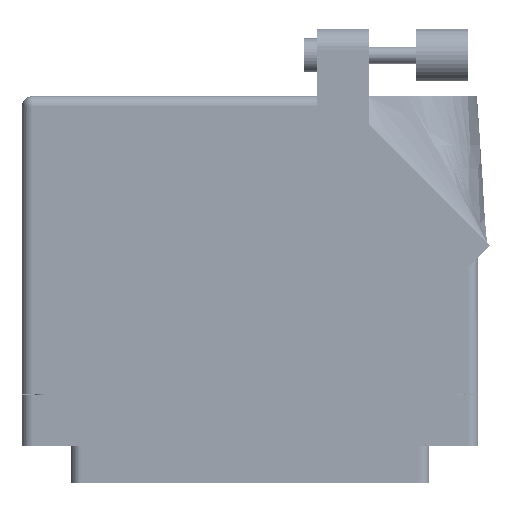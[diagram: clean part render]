
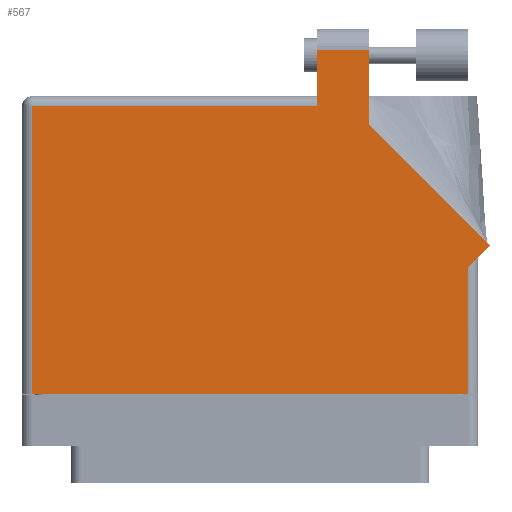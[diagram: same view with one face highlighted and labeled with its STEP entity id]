
A CAD part, front view. The second image highlights one B-rep face of the part: STEP entity #567.
In plain terms, the highlighted face is planar.
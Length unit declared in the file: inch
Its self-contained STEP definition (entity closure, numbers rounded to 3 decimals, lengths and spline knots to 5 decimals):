
#553 = EDGE_CURVE ( 'NONE', #56019, #10716, #7325, .T. ) ;
#567 = ADVANCED_FACE ( 'NONE', ( #53684 ), #71045, .F. ) ;
#1830 = CARTESIAN_POINT ( 'NONE',  ( 1.42971, 0.78571, 0.617 ) ) ;
#5146 = CARTESIAN_POINT ( 'NONE',  ( -1.297, 1.613, 0.617 ) ) ;
#5155 = EDGE_LOOP ( 'NONE', ( #65231, #48399, #29454, #40733, #71744, #52647, #39767, #5816, #29157 ) ) ;
#5320 = VECTOR ( 'NONE', #65843, 39.37008 ) ;
#5524 = VERTEX_POINT ( 'NONE', #60224 ) ;
#5816 = ORIENTED_EDGE ( 'NONE', *, *, #23467, .T. ) ;
#6621 = EDGE_CURVE ( 'NONE', #67285, #56019, #48871, .T. ) ;
#7259 = CARTESIAN_POINT ( 'NONE',  ( -1.297, -0.1, 0.617 ) ) ;
#7325 = LINE ( 'NONE', #70539, #44837 ) ;
#9706 = VECTOR ( 'NONE', #67357, 39.37008 ) ;
#10716 = VERTEX_POINT ( 'NONE', #7259 ) ;
#12158 = DIRECTION ( 'NONE',  ( 1., 0., 0. ) ) ;
#12598 = DIRECTION ( 'NONE',  ( -0.707, 0.707, 0. ) ) ;
#14162 = DIRECTION ( 'NONE',  ( -1., 0., 0. ) ) ;
#14236 = CARTESIAN_POINT ( 'NONE',  ( -1.359, 1.675, 0.617 ) ) ;
#15503 = DIRECTION ( 'NONE',  ( 0., 0., -1. ) ) ;
#15565 = CARTESIAN_POINT ( 'NONE',  ( 0.399, 1.675, 0.617 ) ) ;
#20514 = LINE ( 'NONE', #59876, #5320 ) ;
#20780 = DIRECTION ( 'NONE',  ( 0., -1., 0. ) ) ;
#21946 = AXIS2_PLACEMENT_3D ( 'NONE', #14236, #15503, #73035 ) ;
#23467 = EDGE_CURVE ( 'NONE', #33412, #65912, #20514, .T. ) ;
#24420 = CARTESIAN_POINT ( 'NONE',  ( 1.297, -0.1, 0.617 ) ) ;
#25420 = LINE ( 'NONE', #1830, #34252 ) ;
#26134 = VERTEX_POINT ( 'NONE', #42292 ) ;
#28029 = VECTOR ( 'NONE', #14162, 39.37008 ) ;
#28233 = VECTOR ( 'NONE', #20780, 39.37008 ) ;
#28450 = LINE ( 'NONE', #52500, #62269 ) ;
#29157 = ORIENTED_EDGE ( 'NONE', *, *, #33405, .T. ) ;
#29357 = CARTESIAN_POINT ( 'NONE',  ( 0.706, 1.50942, 0.617 ) ) ;
#29454 = ORIENTED_EDGE ( 'NONE', *, *, #32032, .T. ) ;
#29729 = LINE ( 'NONE', #29357, #51129 ) ;
#31223 = DIRECTION ( 'NONE',  ( 0., -1., 0. ) ) ;
#32032 = EDGE_CURVE ( 'NONE', #44872, #67285, #62049, .T. ) ;
#32400 = CARTESIAN_POINT ( 'NONE',  ( 0.399, 1.613, 0.617 ) ) ;
#32910 = LINE ( 'NONE', #45788, #48856 ) ;
#33076 = CARTESIAN_POINT ( 'NONE',  ( 1.42971, 0.78571, 0.617 ) ) ;
#33405 = EDGE_CURVE ( 'NONE', #65912, #26134, #25420, .T. ) ;
#33412 = VERTEX_POINT ( 'NONE', #70382 ) ;
#33787 = CARTESIAN_POINT ( 'NONE',  ( -1.359, 1.613, 0.617 ) ) ;
#34252 = VECTOR ( 'NONE', #12598, 39.37008 ) ;
#34839 = DIRECTION ( 'NONE',  ( 0., 1., 0. ) ) ;
#36847 = EDGE_CURVE ( 'NONE', #63888, #33412, #28450, .T. ) ;
#39032 = EDGE_CURVE ( 'NONE', #10716, #63888, #32910, .T. ) ;
#39767 = ORIENTED_EDGE ( 'NONE', *, *, #36847, .T. ) ;
#40076 = CARTESIAN_POINT ( 'NONE',  ( 0.399, 1.95, 0.617 ) ) ;
#40733 = ORIENTED_EDGE ( 'NONE', *, *, #6621, .T. ) ;
#42292 = CARTESIAN_POINT ( 'NONE',  ( 0.706, 1.50942, 0.617 ) ) ;
#44083 = LINE ( 'NONE', #54230, #28029 ) ;
#44837 = VECTOR ( 'NONE', #31223, 39.37008 ) ;
#44872 = VERTEX_POINT ( 'NONE', #40076 ) ;
#45788 = CARTESIAN_POINT ( 'NONE',  ( -1.359, -0.1, 0.617 ) ) ;
#46879 = EDGE_CURVE ( 'NONE', #5524, #44872, #44083, .T. ) ;
#47125 = EDGE_CURVE ( 'NONE', #26134, #5524, #29729, .T. ) ;
#48399 = ORIENTED_EDGE ( 'NONE', *, *, #46879, .T. ) ;
#48856 = VECTOR ( 'NONE', #12158, 39.37008 ) ;
#48871 = LINE ( 'NONE', #33787, #9706 ) ;
#51129 = VECTOR ( 'NONE', #34839, 39.37008 ) ;
#52500 = CARTESIAN_POINT ( 'NONE',  ( 1.297, 0.715, 0.617 ) ) ;
#52647 = ORIENTED_EDGE ( 'NONE', *, *, #39032, .T. ) ;
#53254 = DIRECTION ( 'NONE',  ( 0., 1., 0. ) ) ;
#53684 = FACE_OUTER_BOUND ( 'NONE', #5155, .T. ) ;
#54230 = CARTESIAN_POINT ( 'NONE',  ( 0.399, 1.95, 0.617 ) ) ;
#56019 = VERTEX_POINT ( 'NONE', #5146 ) ;
#59876 = CARTESIAN_POINT ( 'NONE',  ( 1.359, 0.715, 0.617 ) ) ;
#60224 = CARTESIAN_POINT ( 'NONE',  ( 0.706, 1.95, 0.617 ) ) ;
#62049 = LINE ( 'NONE', #15565, #28233 ) ;
#62269 = VECTOR ( 'NONE', #53254, 39.37008 ) ;
#63888 = VERTEX_POINT ( 'NONE', #24420 ) ;
#65231 = ORIENTED_EDGE ( 'NONE', *, *, #47125, .T. ) ;
#65843 = DIRECTION ( 'NONE',  ( 0.707, 0.707, 0. ) ) ;
#65912 = VERTEX_POINT ( 'NONE', #33076 ) ;
#67285 = VERTEX_POINT ( 'NONE', #32400 ) ;
#67357 = DIRECTION ( 'NONE',  ( -1., 0., 0. ) ) ;
#70382 = CARTESIAN_POINT ( 'NONE',  ( 1.297, 0.653, 0.617 ) ) ;
#70539 = CARTESIAN_POINT ( 'NONE',  ( -1.297, -0.1, 0.617 ) ) ;
#71045 = PLANE ( 'NONE',  #21946 ) ;
#71744 = ORIENTED_EDGE ( 'NONE', *, *, #553, .T. ) ;
#73035 = DIRECTION ( 'NONE',  ( -1., 0., 0. ) ) ;
